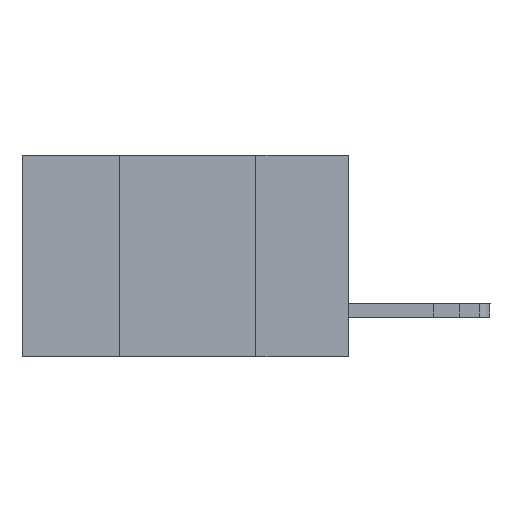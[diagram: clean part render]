
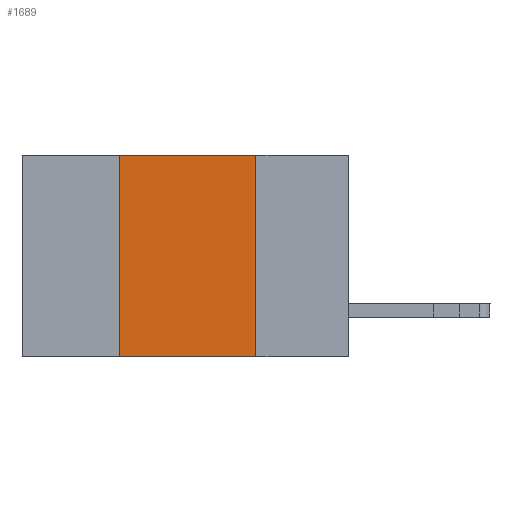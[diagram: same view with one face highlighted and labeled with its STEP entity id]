
A CAD part, left-side view. The second image highlights one B-rep face of the part: STEP entity #1689.
In plain terms, the highlighted planar face has unit normal (-1, 0, 0).
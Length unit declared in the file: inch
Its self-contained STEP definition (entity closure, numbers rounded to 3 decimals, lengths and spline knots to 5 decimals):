
#1143 = CARTESIAN_POINT ( 'NONE',  ( 0., 0.6, 0. ) ) ;
#1689 = ADVANCED_FACE ( 'NONE', ( #11646 ), #15320, .F. ) ;
#1924 = VERTEX_POINT ( 'NONE', #10016 ) ;
#2366 = DIRECTION ( 'NONE',  ( 0., -1., 0. ) ) ;
#2927 = DIRECTION ( 'NONE',  ( 1., 0., 0. ) ) ;
#3993 = DIRECTION ( 'NONE',  ( 0., 0., -1. ) ) ;
#4440 = ORIENTED_EDGE ( 'NONE', *, *, #9346, .F. ) ;
#4699 = VERTEX_POINT ( 'NONE', #11320 ) ;
#4819 = LINE ( 'NONE', #1143, #13223 ) ;
#4954 = EDGE_LOOP ( 'NONE', ( #11399, #4440, #10496, #14012 ) ) ;
#4969 = LINE ( 'NONE', #15239, #7735 ) ;
#5257 = LINE ( 'NONE', #15845, #15924 ) ;
#5459 = DIRECTION ( 'NONE',  ( 0., 0., -1. ) ) ;
#6773 = LINE ( 'NONE', #15553, #10590 ) ;
#7056 = VERTEX_POINT ( 'NONE', #11421 ) ;
#7735 = VECTOR ( 'NONE', #3993, 39.37008 ) ;
#8032 = EDGE_CURVE ( 'NONE', #4699, #1924, #4969, .T. ) ;
#8042 = VERTEX_POINT ( 'NONE', #10180 ) ;
#8141 = EDGE_CURVE ( 'NONE', #8042, #1924, #6773, .T. ) ;
#8417 = DIRECTION ( 'NONE',  ( 0., 0., 1. ) ) ;
#9346 = EDGE_CURVE ( 'NONE', #7056, #4699, #4819, .T. ) ;
#10016 = CARTESIAN_POINT ( 'NONE',  ( 0., 0.17, -0.37 ) ) ;
#10180 = CARTESIAN_POINT ( 'NONE',  ( 0., 0.42, -0.37 ) ) ;
#10496 = ORIENTED_EDGE ( 'NONE', *, *, #13856, .F. ) ;
#10590 = VECTOR ( 'NONE', #12870, 39.37008 ) ;
#11320 = CARTESIAN_POINT ( 'NONE',  ( 0., 0.17, 0. ) ) ;
#11399 = ORIENTED_EDGE ( 'NONE', *, *, #8032, .F. ) ;
#11421 = CARTESIAN_POINT ( 'NONE',  ( 0., 0.42, 0. ) ) ;
#11646 = FACE_OUTER_BOUND ( 'NONE', #4954, .T. ) ;
#12870 = DIRECTION ( 'NONE',  ( 0., -1., 0. ) ) ;
#13223 = VECTOR ( 'NONE', #2366, 39.37008 ) ;
#13856 = EDGE_CURVE ( 'NONE', #8042, #7056, #5257, .T. ) ;
#13868 = AXIS2_PLACEMENT_3D ( 'NONE', #14188, #2927, #5459 ) ;
#14012 = ORIENTED_EDGE ( 'NONE', *, *, #8141, .T. ) ;
#14188 = CARTESIAN_POINT ( 'NONE',  ( 0., 0.6, 0. ) ) ;
#15239 = CARTESIAN_POINT ( 'NONE',  ( 0., 0.17, -0.37 ) ) ;
#15320 = PLANE ( 'NONE',  #13868 ) ;
#15553 = CARTESIAN_POINT ( 'NONE',  ( 0., 0.6, -0.37 ) ) ;
#15845 = CARTESIAN_POINT ( 'NONE',  ( 0., 0.42, -0.37 ) ) ;
#15924 = VECTOR ( 'NONE', #8417, 39.37008 ) ;
